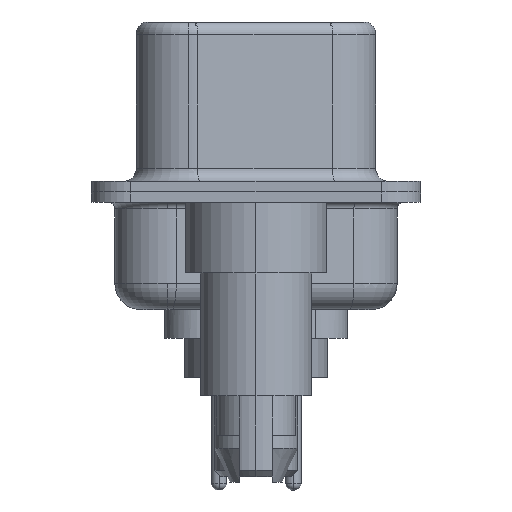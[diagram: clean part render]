
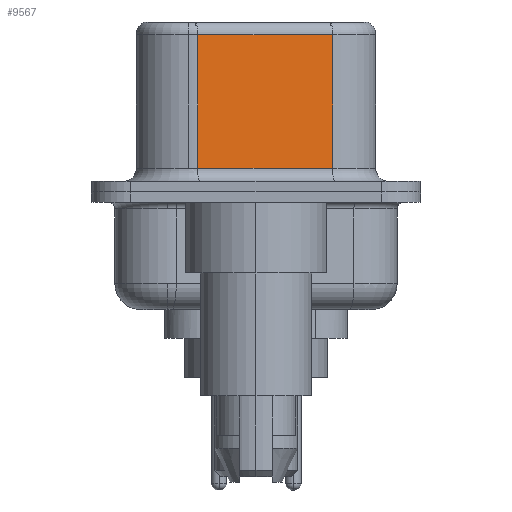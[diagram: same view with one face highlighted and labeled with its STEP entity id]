
A CAD part, left-side view. The second image highlights one B-rep face of the part: STEP entity #9567.
In plain terms, the highlighted planar face has unit normal (-0.985, -0.174, 0).
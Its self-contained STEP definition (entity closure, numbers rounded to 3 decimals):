
#82 = DIRECTION ( 'NONE',  ( 0.174, -0.985, 0. ) ) ;
#217 = DIRECTION ( 'NONE',  ( 0.985, 0.174, 0. ) ) ;
#723 = VERTEX_POINT ( 'NONE', #10836 ) ;
#1823 = EDGE_CURVE ( 'NONE', #723, #17814, #5716, .T. ) ;
#1935 = ORIENTED_EDGE ( 'NONE', *, *, #1823, .T. ) ;
#2041 = EDGE_CURVE ( 'NONE', #7243, #17814, #14595, .T. ) ;
#3901 = EDGE_CURVE ( 'NONE', #14691, #723, #14528, .T. ) ;
#4297 = DIRECTION ( 'NONE',  ( 0., 0., -1. ) ) ;
#4492 = CARTESIAN_POINT ( 'NONE',  ( 4.58, -2.927, 6.02 ) ) ;
#4607 = AXIS2_PLACEMENT_3D ( 'NONE', #8348, #217, #14180 ) ;
#5716 = LINE ( 'NONE', #12446, #13409 ) ;
#6369 = CARTESIAN_POINT ( 'NONE',  ( 4.58, -2.927, 6.02 ) ) ;
#6422 = VECTOR ( 'NONE', #14752, 1000. ) ;
#6442 = EDGE_CURVE ( 'NONE', #7243, #14691, #8381, .T. ) ;
#7243 = VERTEX_POINT ( 'NONE', #4492 ) ;
#8033 = CARTESIAN_POINT ( 'NONE',  ( 3.67, 2.233, 6.02 ) ) ;
#8348 = CARTESIAN_POINT ( 'NONE',  ( 4.58, -2.927, 6.52 ) ) ;
#8381 = LINE ( 'NONE', #6369, #11962 ) ;
#9128 = DIRECTION ( 'NONE',  ( -0.174, 0.985, 0. ) ) ;
#9567 = ADVANCED_FACE ( 'NONE', ( #15712 ), #9759, .F. ) ;
#9759 = PLANE ( 'NONE',  #4607 ) ;
#10836 = CARTESIAN_POINT ( 'NONE',  ( 3.67, 2.233, 0.9 ) ) ;
#11529 = CARTESIAN_POINT ( 'NONE',  ( 4.58, -2.927, 6.52 ) ) ;
#11962 = VECTOR ( 'NONE', #9128, 1000. ) ;
#12446 = CARTESIAN_POINT ( 'NONE',  ( 4.58, -2.927, 0.9 ) ) ;
#13233 = ORIENTED_EDGE ( 'NONE', *, *, #2041, .F. ) ;
#13409 = VECTOR ( 'NONE', #82, 1000. ) ;
#14180 = DIRECTION ( 'NONE',  ( -0.174, 0.985, 0. ) ) ;
#14320 = VECTOR ( 'NONE', #4297, 1000. ) ;
#14323 = CARTESIAN_POINT ( 'NONE',  ( 4.58, -2.927, 0.9 ) ) ;
#14528 = LINE ( 'NONE', #15339, #14320 ) ;
#14595 = LINE ( 'NONE', #11529, #6422 ) ;
#14691 = VERTEX_POINT ( 'NONE', #8033 ) ;
#14752 = DIRECTION ( 'NONE',  ( 0., 0., -1. ) ) ;
#15339 = CARTESIAN_POINT ( 'NONE',  ( 3.67, 2.233, 6.52 ) ) ;
#15698 = EDGE_LOOP ( 'NONE', ( #13233, #15751, #16994, #1935 ) ) ;
#15712 = FACE_OUTER_BOUND ( 'NONE', #15698, .T. ) ;
#15751 = ORIENTED_EDGE ( 'NONE', *, *, #6442, .T. ) ;
#16994 = ORIENTED_EDGE ( 'NONE', *, *, #3901, .T. ) ;
#17814 = VERTEX_POINT ( 'NONE', #14323 ) ;
